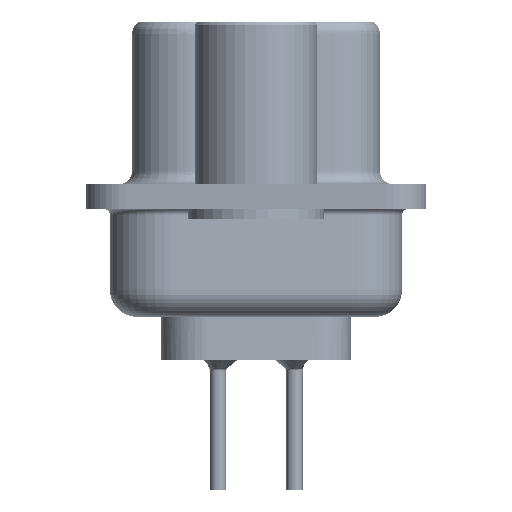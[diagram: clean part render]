
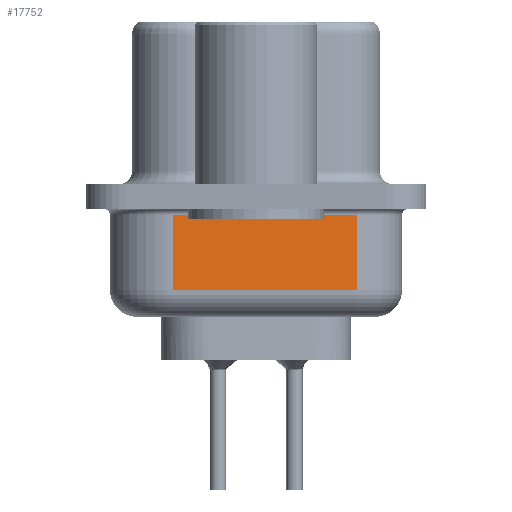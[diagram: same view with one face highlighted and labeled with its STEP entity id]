
A CAD part, left-side view. The second image highlights one B-rep face of the part: STEP entity #17752.
In plain terms, the highlighted planar face has unit normal (-0.985, -0.174, 0).
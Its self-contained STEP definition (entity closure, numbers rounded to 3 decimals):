
#212 = EDGE_CURVE ( 'NONE', #16242, #25293, #30051, .T. ) ;
#260 = CARTESIAN_POINT ( 'NONE',  ( 2.88, 3.053, -3.45 ) ) ;
#3568 = EDGE_CURVE ( 'NONE', #14238, #16242, #24358, .T. ) ;
#4398 = LINE ( 'NONE', #23097, #16165 ) ;
#5503 = CARTESIAN_POINT ( 'NONE',  ( 2.88, 3.053, -4.45 ) ) ;
#6196 = ORIENTED_EDGE ( 'NONE', *, *, #212, .T. ) ;
#8412 = EDGE_CURVE ( 'NONE', #25293, #19673, #18617, .T. ) ;
#12570 = DIRECTION ( 'NONE',  ( 0.174, -0.985, 0. ) ) ;
#13597 = DIRECTION ( 'NONE',  ( 0., 0., 1. ) ) ;
#13793 = VECTOR ( 'NONE', #18917, 1000. ) ;
#14238 = VERTEX_POINT ( 'NONE', #260 ) ;
#14851 = DIRECTION ( 'NONE',  ( 0.985, 0.174, 0. ) ) ;
#14993 = ORIENTED_EDGE ( 'NONE', *, *, #17918, .F. ) ;
#15395 = ORIENTED_EDGE ( 'NONE', *, *, #8412, .T. ) ;
#16165 = VECTOR ( 'NONE', #13597, 1000. ) ;
#16242 = VERTEX_POINT ( 'NONE', #27705 ) ;
#16408 = DIRECTION ( 'NONE',  ( 0., 0., 1. ) ) ;
#16815 = VECTOR ( 'NONE', #16408, 1000. ) ;
#17150 = CARTESIAN_POINT ( 'NONE',  ( 2.88, 3.053, -3.45 ) ) ;
#17752 = ADVANCED_FACE ( 'NONE', ( #26169 ), #24042, .F. ) ;
#17918 = EDGE_CURVE ( 'NONE', #14238, #19673, #4398, .T. ) ;
#17933 = VECTOR ( 'NONE', #12570, 1000. ) ;
#18617 = LINE ( 'NONE', #27948, #13793 ) ;
#18917 = DIRECTION ( 'NONE',  ( -0.174, 0.985, 0. ) ) ;
#19673 = VERTEX_POINT ( 'NONE', #25429 ) ;
#20530 = CARTESIAN_POINT ( 'NONE',  ( 4.079, -3.747, -0.7 ) ) ;
#23097 = CARTESIAN_POINT ( 'NONE',  ( 2.88, 3.053, -4.45 ) ) ;
#24042 = PLANE ( 'NONE',  #24991 ) ;
#24200 = DIRECTION ( 'NONE',  ( -0.174, 0.985, 0. ) ) ;
#24358 = LINE ( 'NONE', #17150, #17933 ) ;
#24991 = AXIS2_PLACEMENT_3D ( 'NONE', #5503, #14851, #24200 ) ;
#25293 = VERTEX_POINT ( 'NONE', #20530 ) ;
#25429 = CARTESIAN_POINT ( 'NONE',  ( 2.88, 3.053, -0.7 ) ) ;
#25898 = EDGE_LOOP ( 'NONE', ( #14993, #28363, #6196, #15395 ) ) ;
#26169 = FACE_OUTER_BOUND ( 'NONE', #25898, .T. ) ;
#27705 = CARTESIAN_POINT ( 'NONE',  ( 4.079, -3.747, -3.45 ) ) ;
#27901 = CARTESIAN_POINT ( 'NONE',  ( 4.079, -3.747, -4.45 ) ) ;
#27948 = CARTESIAN_POINT ( 'NONE',  ( 2.88, 3.053, -0.7 ) ) ;
#28363 = ORIENTED_EDGE ( 'NONE', *, *, #3568, .T. ) ;
#30051 = LINE ( 'NONE', #27901, #16815 ) ;
